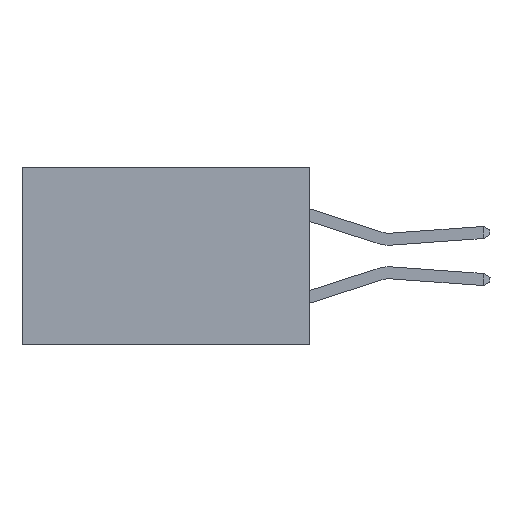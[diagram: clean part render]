
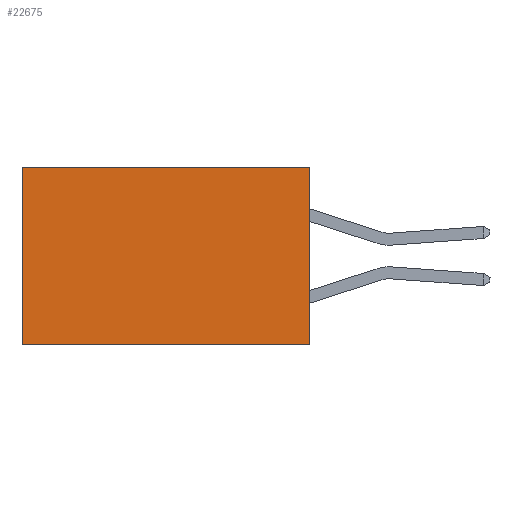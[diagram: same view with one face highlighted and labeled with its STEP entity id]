
A CAD part, left-side view. The second image highlights one B-rep face of the part: STEP entity #22675.
In plain terms, the highlighted planar face has unit normal (-1, 0, 0).
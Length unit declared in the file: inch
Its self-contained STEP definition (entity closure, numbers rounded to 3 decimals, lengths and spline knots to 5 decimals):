
#255 = PLANE ( 'NONE',  #14293 ) ;
#1517 = ORIENTED_EDGE ( 'NONE', *, *, #6816, .F. ) ;
#2305 = DIRECTION ( 'NONE',  ( 0., 0., -1. ) ) ;
#3024 = CARTESIAN_POINT ( 'NONE',  ( 0.298, 0.6, 0. ) ) ;
#3266 = VERTEX_POINT ( 'NONE', #3024 ) ;
#3418 = CARTESIAN_POINT ( 'NONE',  ( 0.298, 0., -0.37 ) ) ;
#4620 = EDGE_CURVE ( 'NONE', #14163, #3266, #4944, .T. ) ;
#4944 = LINE ( 'NONE', #8872, #7302 ) ;
#5586 = CARTESIAN_POINT ( 'NONE',  ( 0.298, 0., -0.37 ) ) ;
#5844 = DIRECTION ( 'NONE',  ( 1., 0., 0. ) ) ;
#6816 = EDGE_CURVE ( 'NONE', #9197, #12260, #23887, .T. ) ;
#7140 = ORIENTED_EDGE ( 'NONE', *, *, #22155, .T. ) ;
#7302 = VECTOR ( 'NONE', #10614, 39.37008 ) ;
#7594 = CARTESIAN_POINT ( 'NONE',  ( 0.298, 0., 0. ) ) ;
#8872 = CARTESIAN_POINT ( 'NONE',  ( 0.298, 0., 0. ) ) ;
#9197 = VERTEX_POINT ( 'NONE', #5586 ) ;
#9283 = LINE ( 'NONE', #21103, #13118 ) ;
#9325 = ORIENTED_EDGE ( 'NONE', *, *, #16653, .F. ) ;
#10614 = DIRECTION ( 'NONE',  ( 0., 1., 0. ) ) ;
#10722 = VECTOR ( 'NONE', #24428, 39.37008 ) ;
#10973 = CARTESIAN_POINT ( 'NONE',  ( 0.298, 0.6, 0. ) ) ;
#11915 = LINE ( 'NONE', #10973, #10722 ) ;
#12260 = VERTEX_POINT ( 'NONE', #19580 ) ;
#13118 = VECTOR ( 'NONE', #2305, 39.37008 ) ;
#14163 = VERTEX_POINT ( 'NONE', #15394 ) ;
#14293 = AXIS2_PLACEMENT_3D ( 'NONE', #7594, #5844, #20896 ) ;
#15394 = CARTESIAN_POINT ( 'NONE',  ( 0.298, 0., 0. ) ) ;
#16064 = FACE_OUTER_BOUND ( 'NONE', #19099, .T. ) ;
#16653 = EDGE_CURVE ( 'NONE', #14163, #9197, #9283, .T. ) ;
#19099 = EDGE_LOOP ( 'NONE', ( #7140, #1517, #9325, #23181 ) ) ;
#19580 = CARTESIAN_POINT ( 'NONE',  ( 0.298, 0.6, -0.37 ) ) ;
#20437 = DIRECTION ( 'NONE',  ( 0., 1., 0. ) ) ;
#20896 = DIRECTION ( 'NONE',  ( 0., 0., -1. ) ) ;
#21103 = CARTESIAN_POINT ( 'NONE',  ( 0.298, 0., 0. ) ) ;
#22155 = EDGE_CURVE ( 'NONE', #3266, #12260, #11915, .T. ) ;
#22675 = ADVANCED_FACE ( 'NONE', ( #16064 ), #255, .F. ) ;
#23001 = VECTOR ( 'NONE', #20437, 39.37008 ) ;
#23181 = ORIENTED_EDGE ( 'NONE', *, *, #4620, .T. ) ;
#23887 = LINE ( 'NONE', #3418, #23001 ) ;
#24428 = DIRECTION ( 'NONE',  ( 0., 0., -1. ) ) ;
